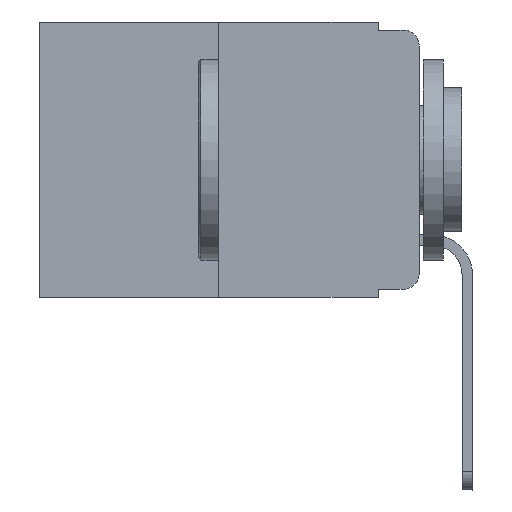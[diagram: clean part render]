
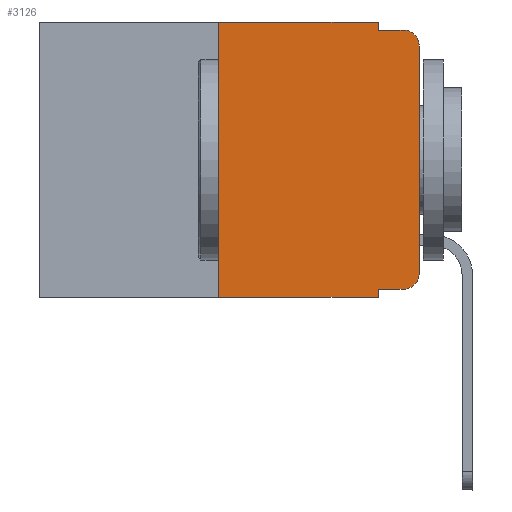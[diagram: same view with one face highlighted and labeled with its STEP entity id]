
A CAD part, left-side view. The second image highlights one B-rep face of the part: STEP entity #3126.
In plain terms, the highlighted planar face has unit normal (-1, 0, 0).
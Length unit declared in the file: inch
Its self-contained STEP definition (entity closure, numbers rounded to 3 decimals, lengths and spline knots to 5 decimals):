
#41 = CARTESIAN_POINT ( 'NONE',  ( 0., 0.051, -0.333 ) ) ;
#491 = EDGE_CURVE ( 'NONE', #10106, #10271, #12112, .T. ) ;
#624 = LINE ( 'NONE', #5545, #7377 ) ;
#1079 = VERTEX_POINT ( 'NONE', #12924 ) ;
#1223 = VECTOR ( 'NONE', #1883, 39.37008 ) ;
#1292 = EDGE_CURVE ( 'NONE', #14348, #6826, #11070, .T. ) ;
#1297 = CARTESIAN_POINT ( 'NONE',  ( 0., 0., -0.03 ) ) ;
#1863 = ORIENTED_EDGE ( 'NONE', *, *, #7754, .T. ) ;
#1883 = DIRECTION ( 'NONE',  ( 0., -1., 0. ) ) ;
#2026 = CIRCLE ( 'NONE', #10591, 0.02 ) ;
#2076 = VERTEX_POINT ( 'NONE', #1297 ) ;
#2421 = VECTOR ( 'NONE', #11095, 39.37008 ) ;
#2629 = CARTESIAN_POINT ( 'NONE',  ( 0., 0.02, -0.01 ) ) ;
#2955 = EDGE_CURVE ( 'NONE', #11117, #2076, #624, .T. ) ;
#3126 = ADVANCED_FACE ( 'NONE', ( #12737 ), #5769, .F. ) ;
#3672 = CARTESIAN_POINT ( 'NONE',  ( 0., 0.473, 0. ) ) ;
#3838 = ORIENTED_EDGE ( 'NONE', *, *, #2955, .T. ) ;
#5057 = EDGE_CURVE ( 'NONE', #9698, #6223, #5632, .T. ) ;
#5230 = DIRECTION ( 'NONE',  ( 0., -1., 0. ) ) ;
#5545 = CARTESIAN_POINT ( 'NONE',  ( 0., 0., 0. ) ) ;
#5632 = LINE ( 'NONE', #10295, #11327 ) ;
#5698 = ORIENTED_EDGE ( 'NONE', *, *, #13145, .T. ) ;
#5769 = PLANE ( 'NONE',  #7647 ) ;
#5771 = DIRECTION ( 'NONE',  ( 0., 0., -1. ) ) ;
#5885 = CARTESIAN_POINT ( 'NONE',  ( 0., 0.051, 0. ) ) ;
#6223 = VERTEX_POINT ( 'NONE', #11217 ) ;
#6671 = ORIENTED_EDGE ( 'NONE', *, *, #491, .F. ) ;
#6712 = ORIENTED_EDGE ( 'NONE', *, *, #14258, .F. ) ;
#6826 = VERTEX_POINT ( 'NONE', #8069 ) ;
#7074 = DIRECTION ( 'NONE',  ( 1., 0., 0. ) ) ;
#7377 = VECTOR ( 'NONE', #7702, 39.37008 ) ;
#7517 = ORIENTED_EDGE ( 'NONE', *, *, #5057, .F. ) ;
#7647 = AXIS2_PLACEMENT_3D ( 'NONE', #8154, #7074, #9145 ) ;
#7702 = DIRECTION ( 'NONE',  ( 0., 0., 1. ) ) ;
#7754 = EDGE_CURVE ( 'NONE', #14348, #6223, #7886, .T. ) ;
#7886 = LINE ( 'NONE', #12388, #1223 ) ;
#8036 = CARTESIAN_POINT ( 'NONE',  ( 0., 0.02, -0.03 ) ) ;
#8062 = VECTOR ( 'NONE', #11696, 39.37008 ) ;
#8069 = CARTESIAN_POINT ( 'NONE',  ( 0., 0.25, 0. ) ) ;
#8089 = CARTESIAN_POINT ( 'NONE',  ( 0., 0.051, 0. ) ) ;
#8154 = CARTESIAN_POINT ( 'NONE',  ( 0., 0.473, 0. ) ) ;
#8261 = EDGE_CURVE ( 'NONE', #9698, #1079, #13381, .T. ) ;
#8522 = CARTESIAN_POINT ( 'NONE',  ( 0., 0.25, -0.343 ) ) ;
#8680 = CARTESIAN_POINT ( 'NONE',  ( 0., 0.051, -0.01 ) ) ;
#8728 = CARTESIAN_POINT ( 'NONE',  ( 0., 0.051, -0.333 ) ) ;
#8778 = EDGE_CURVE ( 'NONE', #1079, #11117, #9552, .T. ) ;
#9145 = DIRECTION ( 'NONE',  ( 0., 0., -1. ) ) ;
#9405 = CARTESIAN_POINT ( 'NONE',  ( 0., 0.051, -0.01 ) ) ;
#9521 = DIRECTION ( 'NONE',  ( 0., -1., 0. ) ) ;
#9525 = DIRECTION ( 'NONE',  ( -1., 0., 0. ) ) ;
#9552 = CIRCLE ( 'NONE', #14919, 0.02 ) ;
#9623 = EDGE_CURVE ( 'NONE', #12283, #10106, #13838, .T. ) ;
#9698 = VERTEX_POINT ( 'NONE', #41 ) ;
#10106 = VERTEX_POINT ( 'NONE', #9405 ) ;
#10226 = CARTESIAN_POINT ( 'NONE',  ( 0., 0.25, 0. ) ) ;
#10271 = VERTEX_POINT ( 'NONE', #2629 ) ;
#10295 = CARTESIAN_POINT ( 'NONE',  ( 0., 0.051, 0. ) ) ;
#10591 = AXIS2_PLACEMENT_3D ( 'NONE', #8036, #11691, #13751 ) ;
#10655 = LINE ( 'NONE', #3672, #11641 ) ;
#11017 = EDGE_LOOP ( 'NONE', ( #3838, #5698, #6671, #13631, #6712, #14904, #1863, #7517, #13033, #12072 ) ) ;
#11070 = LINE ( 'NONE', #10226, #14005 ) ;
#11095 = DIRECTION ( 'NONE',  ( 0., -1., 0. ) ) ;
#11117 = VERTEX_POINT ( 'NONE', #13590 ) ;
#11217 = CARTESIAN_POINT ( 'NONE',  ( 0., 0.051, -0.343 ) ) ;
#11218 = DIRECTION ( 'NONE',  ( 0., 0., 1. ) ) ;
#11327 = VECTOR ( 'NONE', #11360, 39.37008 ) ;
#11360 = DIRECTION ( 'NONE',  ( 0., 0., -1. ) ) ;
#11641 = VECTOR ( 'NONE', #9521, 39.37008 ) ;
#11691 = DIRECTION ( 'NONE',  ( -1., 0., 0. ) ) ;
#11696 = DIRECTION ( 'NONE',  ( 0., 0., -1. ) ) ;
#12072 = ORIENTED_EDGE ( 'NONE', *, *, #8778, .T. ) ;
#12112 = LINE ( 'NONE', #8680, #14298 ) ;
#12283 = VERTEX_POINT ( 'NONE', #8089 ) ;
#12388 = CARTESIAN_POINT ( 'NONE',  ( 0., 0.473, -0.343 ) ) ;
#12737 = FACE_OUTER_BOUND ( 'NONE', #11017, .T. ) ;
#12924 = CARTESIAN_POINT ( 'NONE',  ( 0., 0.02, -0.333 ) ) ;
#13033 = ORIENTED_EDGE ( 'NONE', *, *, #8261, .T. ) ;
#13145 = EDGE_CURVE ( 'NONE', #2076, #10271, #2026, .T. ) ;
#13381 = LINE ( 'NONE', #8728, #2421 ) ;
#13590 = CARTESIAN_POINT ( 'NONE',  ( 0., 0., -0.313 ) ) ;
#13631 = ORIENTED_EDGE ( 'NONE', *, *, #9623, .F. ) ;
#13751 = DIRECTION ( 'NONE',  ( 0., 0., -1. ) ) ;
#13838 = LINE ( 'NONE', #5885, #8062 ) ;
#14005 = VECTOR ( 'NONE', #11218, 39.37008 ) ;
#14103 = CARTESIAN_POINT ( 'NONE',  ( 0., 0.02, -0.313 ) ) ;
#14258 = EDGE_CURVE ( 'NONE', #6826, #12283, #10655, .T. ) ;
#14298 = VECTOR ( 'NONE', #5230, 39.37008 ) ;
#14348 = VERTEX_POINT ( 'NONE', #8522 ) ;
#14904 = ORIENTED_EDGE ( 'NONE', *, *, #1292, .F. ) ;
#14919 = AXIS2_PLACEMENT_3D ( 'NONE', #14103, #9525, #5771 ) ;
